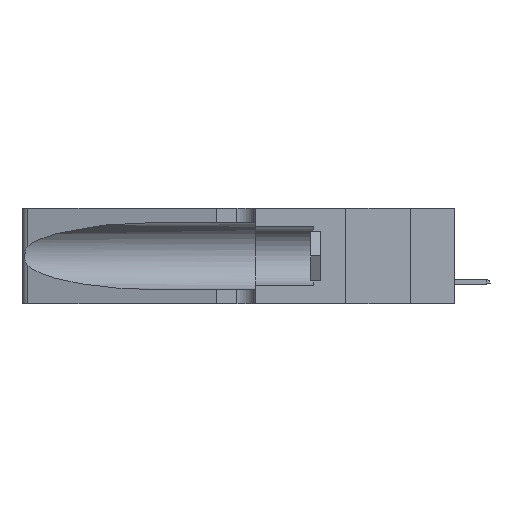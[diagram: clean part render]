
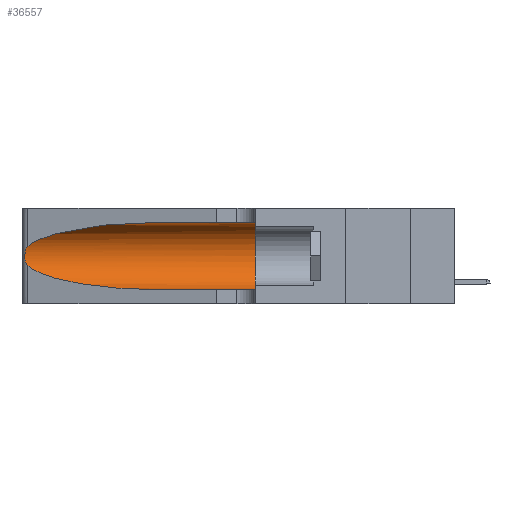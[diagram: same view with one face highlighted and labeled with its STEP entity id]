
A CAD part, left-side view. The second image highlights one B-rep face of the part: STEP entity #36557.
In plain terms, the highlighted cylindrical face has radius 3.308 mm (diameter 6.617 mm), a partial arc.
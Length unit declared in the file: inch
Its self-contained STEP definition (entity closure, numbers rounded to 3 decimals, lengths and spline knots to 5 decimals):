
#967 = EDGE_CURVE ( 'NONE', #26376, #7610, #4779, .T. ) ;
#2240 = CARTESIAN_POINT ( 'NONE',  ( 0.25487, 1.22718, 0.22369 ) ) ;
#3422 = CARTESIAN_POINT ( 'NONE',  ( 0.1305, 0.72297, 0.31525 ) ) ;
#4674 = CARTESIAN_POINT ( 'NONE',  ( 0.1305, 0.72297, 0.05475 ) ) ;
#4779 =( BOUNDED_CURVE ( )  B_SPLINE_CURVE ( 3, ( #3422, #17767, #32466, #36082 ),
 .UNSPECIFIED., .F., .T. ) 
 B_SPLINE_CURVE_WITH_KNOTS ( ( 4, 4 ),
 ( 1.5708, 2.84003 ),
 .UNSPECIFIED. ) 
 CURVE ( )  GEOMETRIC_REPRESENTATION_ITEM ( )  RATIONAL_B_SPLINE_CURVE ( ( 1., 0.87, 0.87, 1. ) ) 
 REPRESENTATION_ITEM ( '' )  );
#5564 = DIRECTION ( 'NONE',  ( 0., -1., 0. ) ) ;
#7097 = VECTOR ( 'NONE', #25426, 39.37008 ) ;
#7477 = DIRECTION ( 'NONE',  ( 0., 1., 0. ) ) ;
#7610 = VERTEX_POINT ( 'NONE', #12997 ) ;
#8025 = VERTEX_POINT ( 'NONE', #32963 ) ;
#8377 = EDGE_CURVE ( 'NONE', #26376, #26798, #17221, .T. ) ;
#8524 = CARTESIAN_POINT ( 'NONE',  ( 0.26017, 1.23833, 0.17102 ) ) ;
#8608 = DIRECTION ( 'NONE',  ( 0., 0., -1. ) ) ;
#9209 = EDGE_CURVE ( 'NONE', #7610, #8025, #20982, .T. ) ;
#9583 = ORIENTED_EDGE ( 'NONE', *, *, #26166, .T. ) ;
#9898 = EDGE_CURVE ( 'NONE', #8025, #36270, #21628, .T. ) ;
#10339 = ORIENTED_EDGE ( 'NONE', *, *, #9898, .T. ) ;
#10750 = CIRCLE ( 'NONE', #29673, 0.13025 ) ;
#11203 = CARTESIAN_POINT ( 'NONE',  ( 0.25639, 1.23184, 0.21858 ) ) ;
#12997 = CARTESIAN_POINT ( 'NONE',  ( 0.25487, 1.22718, 0.22369 ) ) ;
#13537 = LINE ( 'NONE', #16208, #31240 ) ;
#14082 = CARTESIAN_POINT ( 'NONE',  ( 0.26018, 1.23835, 0.19895 ) ) ;
#14442 = CARTESIAN_POINT ( 'NONE',  ( 0.26075, 1.23896, 0.178 ) ) ;
#15777 = EDGE_CURVE ( 'NONE', #26798, #31701, #10750, .T. ) ;
#16127 = CARTESIAN_POINT ( 'NONE',  ( 0.1305, 0.72297, 0.31525 ) ) ;
#16208 = CARTESIAN_POINT ( 'NONE',  ( 0.1305, 1.61858, 0.05475 ) ) ;
#16288 = DIRECTION ( 'NONE',  ( 0., 0., 1. ) ) ;
#16470 = EDGE_LOOP ( 'NONE', ( #18779, #36348, #10339, #9583, #35596, #34358 ) ) ;
#16581 = CARTESIAN_POINT ( 'NONE',  ( 0.25555, 1.22993, 0.14849 ) ) ;
#17221 = LINE ( 'NONE', #34049, #7097 ) ;
#17767 = CARTESIAN_POINT ( 'NONE',  ( 0.18966, 0.96281, 0.31525 ) ) ;
#18779 = ORIENTED_EDGE ( 'NONE', *, *, #967, .T. ) ;
#19050 = CARTESIAN_POINT ( 'NONE',  ( 0.2373, 1.15595, 0.08982 ) ) ;
#20982 = B_SPLINE_CURVE_WITH_KNOTS ( 'NONE', 3,
 ( #2240, #28774, #11203, #34878, #31830, #14082, #22834, #14442, #8524, #28406, #34140, #36978, #16581, #28229 ),
 .UNSPECIFIED., .F., .F.,
 ( 4, 2, 2, 2, 2, 2, 4 ),
 ( 0., 0.00027, 0.00053, 0.00107, 0.0016, 0.00187, 0.00214 ),
 .UNSPECIFIED. ) ;
#21628 =( BOUNDED_CURVE ( )  B_SPLINE_CURVE ( 3, ( #28213, #19050, #30668, #4674 ),
 .UNSPECIFIED., .F., .T. ) 
 B_SPLINE_CURVE_WITH_KNOTS ( ( 4, 4 ),
 ( 3.44316, 4.71239 ),
 .UNSPECIFIED. ) 
 CURVE ( )  GEOMETRIC_REPRESENTATION_ITEM ( )  RATIONAL_B_SPLINE_CURVE ( ( 1., 0.87, 0.87, 1. ) ) 
 REPRESENTATION_ITEM ( '' )  );
#22008 = CARTESIAN_POINT ( 'NONE',  ( 0.1305, 0.35, 0.185 ) ) ;
#22834 = CARTESIAN_POINT ( 'NONE',  ( 0.26075, 1.23896, 0.19203 ) ) ;
#24091 = CARTESIAN_POINT ( 'NONE',  ( 0.1305, 0.72297, 0.05475 ) ) ;
#25426 = DIRECTION ( 'NONE',  ( 0., -1., 0. ) ) ;
#25608 = AXIS2_PLACEMENT_3D ( 'NONE', #25780, #5564, #8608 ) ;
#25619 = CARTESIAN_POINT ( 'NONE',  ( 0.1305, 0.35, 0.05475 ) ) ;
#25780 = CARTESIAN_POINT ( 'NONE',  ( 0.1305, 1.61858, 0.185 ) ) ;
#26166 = EDGE_CURVE ( 'NONE', #36270, #31701, #13537, .T. ) ;
#26376 = VERTEX_POINT ( 'NONE', #16127 ) ;
#26798 = VERTEX_POINT ( 'NONE', #28877 ) ;
#28213 = CARTESIAN_POINT ( 'NONE',  ( 0.25487, 1.22718, 0.14631 ) ) ;
#28229 = CARTESIAN_POINT ( 'NONE',  ( 0.25487, 1.22718, 0.14631 ) ) ;
#28406 = CARTESIAN_POINT ( 'NONE',  ( 0.25856, 1.23593, 0.16098 ) ) ;
#28774 = CARTESIAN_POINT ( 'NONE',  ( 0.25555, 1.22994, 0.2215 ) ) ;
#28877 = CARTESIAN_POINT ( 'NONE',  ( 0.1305, 0.35, 0.31525 ) ) ;
#29673 = AXIS2_PLACEMENT_3D ( 'NONE', #22008, #7477, #16288 ) ;
#30668 = CARTESIAN_POINT ( 'NONE',  ( 0.18966, 0.96281, 0.05475 ) ) ;
#31240 = VECTOR ( 'NONE', #36805, 39.37008 ) ;
#31701 = VERTEX_POINT ( 'NONE', #25619 ) ;
#31732 = CYLINDRICAL_SURFACE ( 'NONE', #25608, 0.13025 ) ;
#31830 = CARTESIAN_POINT ( 'NONE',  ( 0.25854, 1.2359, 0.20912 ) ) ;
#32466 = CARTESIAN_POINT ( 'NONE',  ( 0.2373, 1.15595, 0.28018 ) ) ;
#32963 = CARTESIAN_POINT ( 'NONE',  ( 0.25487, 1.22718, 0.14631 ) ) ;
#34049 = CARTESIAN_POINT ( 'NONE',  ( 0.1305, 1.61858, 0.31525 ) ) ;
#34140 = CARTESIAN_POINT ( 'NONE',  ( 0.25789, 1.23486, 0.15765 ) ) ;
#34358 = ORIENTED_EDGE ( 'NONE', *, *, #8377, .F. ) ;
#34878 = CARTESIAN_POINT ( 'NONE',  ( 0.25787, 1.23484, 0.2124 ) ) ;
#35596 = ORIENTED_EDGE ( 'NONE', *, *, #15777, .F. ) ;
#36082 = CARTESIAN_POINT ( 'NONE',  ( 0.25487, 1.22718, 0.22369 ) ) ;
#36270 = VERTEX_POINT ( 'NONE', #24091 ) ;
#36348 = ORIENTED_EDGE ( 'NONE', *, *, #9209, .T. ) ;
#36557 = ADVANCED_FACE ( 'NONE', ( #37626 ), #31732, .F. ) ;
#36805 = DIRECTION ( 'NONE',  ( 0., -1., 0. ) ) ;
#36978 = CARTESIAN_POINT ( 'NONE',  ( 0.25639, 1.23186, 0.15144 ) ) ;
#37626 = FACE_OUTER_BOUND ( 'NONE', #16470, .T. ) ;
